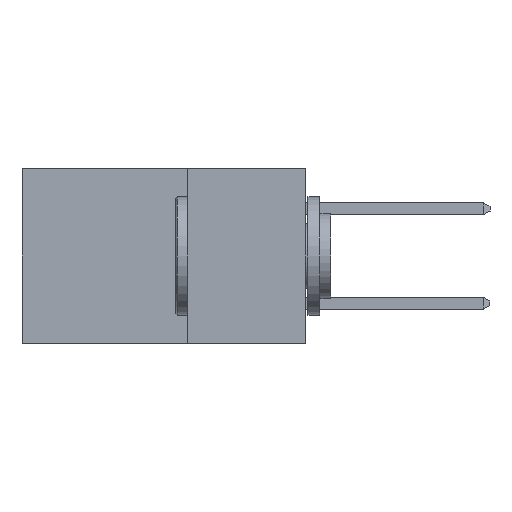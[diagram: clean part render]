
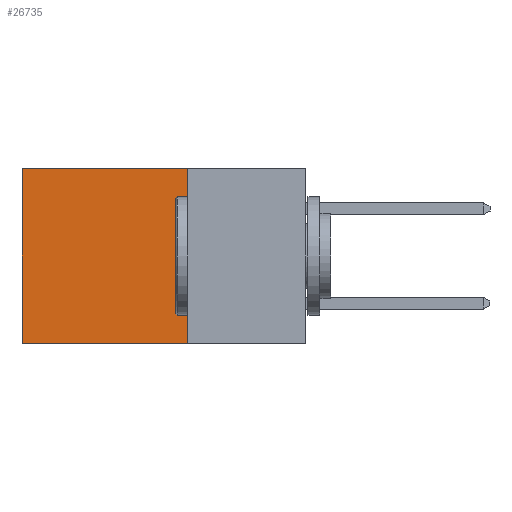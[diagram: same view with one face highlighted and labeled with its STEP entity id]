
A CAD part, left-side view. The second image highlights one B-rep face of the part: STEP entity #26735.
In plain terms, the highlighted planar face has unit normal (-1, 0, 0).
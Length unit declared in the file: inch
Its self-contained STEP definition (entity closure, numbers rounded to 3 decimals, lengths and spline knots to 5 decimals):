
#304 = LINE ( 'NONE', #9937, #19065 ) ;
#713 = VERTEX_POINT ( 'NONE', #22914 ) ;
#761 = DIRECTION ( 'NONE',  ( 0., 1., 0. ) ) ;
#1867 = ORIENTED_EDGE ( 'NONE', *, *, #15210, .F. ) ;
#3820 = LINE ( 'NONE', #6722, #15560 ) ;
#4540 = ORIENTED_EDGE ( 'NONE', *, *, #11922, .F. ) ;
#6082 = FACE_OUTER_BOUND ( 'NONE', #16486, .T. ) ;
#6197 = LINE ( 'NONE', #28611, #29946 ) ;
#6637 = VERTEX_POINT ( 'NONE', #13041 ) ;
#6722 = CARTESIAN_POINT ( 'NONE',  ( 0.298, 0.25, 0. ) ) ;
#8269 = PLANE ( 'NONE',  #22510 ) ;
#9088 = DIRECTION ( 'NONE',  ( 0., 0., -1. ) ) ;
#9231 = DIRECTION ( 'NONE',  ( 0., 0., -1. ) ) ;
#9937 = CARTESIAN_POINT ( 'NONE',  ( 0.298, 0.25, 0. ) ) ;
#11526 = ORIENTED_EDGE ( 'NONE', *, *, #19711, .T. ) ;
#11922 = EDGE_CURVE ( 'NONE', #27301, #6637, #3820, .T. ) ;
#12318 = DIRECTION ( 'NONE',  ( 0., 1., 0. ) ) ;
#13014 = DIRECTION ( 'NONE',  ( 1., 0., 0. ) ) ;
#13041 = CARTESIAN_POINT ( 'NONE',  ( 0.298, 0.25, -0.37 ) ) ;
#14419 = LINE ( 'NONE', #27654, #20539 ) ;
#15210 = EDGE_CURVE ( 'NONE', #6637, #21047, #6197, .T. ) ;
#15560 = VECTOR ( 'NONE', #9088, 39.37008 ) ;
#16486 = EDGE_LOOP ( 'NONE', ( #11526, #1867, #4540, #20679 ) ) ;
#16973 = CARTESIAN_POINT ( 'NONE',  ( 0.298, 0.6, -0.37 ) ) ;
#19065 = VECTOR ( 'NONE', #12318, 39.37008 ) ;
#19711 = EDGE_CURVE ( 'NONE', #713, #21047, #14419, .T. ) ;
#20539 = VECTOR ( 'NONE', #9231, 39.37008 ) ;
#20679 = ORIENTED_EDGE ( 'NONE', *, *, #21022, .T. ) ;
#21022 = EDGE_CURVE ( 'NONE', #27301, #713, #304, .T. ) ;
#21047 = VERTEX_POINT ( 'NONE', #16973 ) ;
#22510 = AXIS2_PLACEMENT_3D ( 'NONE', #26734, #13014, #29007 ) ;
#22914 = CARTESIAN_POINT ( 'NONE',  ( 0.298, 0.6, 0. ) ) ;
#26734 = CARTESIAN_POINT ( 'NONE',  ( 0.298, 0.25, 0. ) ) ;
#26735 = ADVANCED_FACE ( 'NONE', ( #6082 ), #8269, .F. ) ;
#27301 = VERTEX_POINT ( 'NONE', #28679 ) ;
#27654 = CARTESIAN_POINT ( 'NONE',  ( 0.298, 0.6, 0. ) ) ;
#28611 = CARTESIAN_POINT ( 'NONE',  ( 0.298, 0.25, -0.37 ) ) ;
#28679 = CARTESIAN_POINT ( 'NONE',  ( 0.298, 0.25, 0. ) ) ;
#29007 = DIRECTION ( 'NONE',  ( 0., 0., -1. ) ) ;
#29946 = VECTOR ( 'NONE', #761, 39.37008 ) ;
